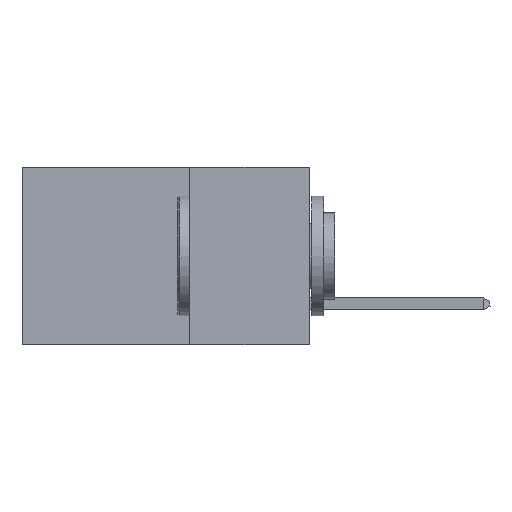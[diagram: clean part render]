
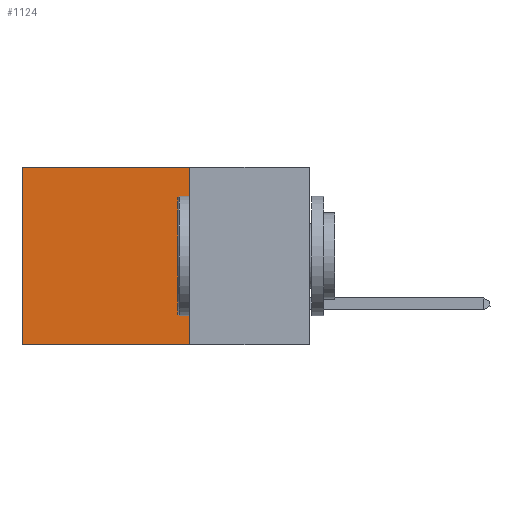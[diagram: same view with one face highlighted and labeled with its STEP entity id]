
A CAD part, left-side view. The second image highlights one B-rep face of the part: STEP entity #1124.
In plain terms, the highlighted planar face has unit normal (-1, 0, 0).
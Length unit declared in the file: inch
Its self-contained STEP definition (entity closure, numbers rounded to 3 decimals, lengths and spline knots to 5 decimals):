
#307 = DIRECTION ( 'NONE',  ( 0., 0., -1. ) ) ;
#353 = EDGE_LOOP ( 'NONE', ( #11530, #10782, #11792, #6361 ) ) ;
#507 = LINE ( 'NONE', #11734, #7460 ) ;
#599 = VERTEX_POINT ( 'NONE', #2296 ) ;
#955 = EDGE_CURVE ( 'NONE', #12459, #10195, #2803, .T. ) ;
#1124 = ADVANCED_FACE ( 'NONE', ( #12735 ), #9657, .F. ) ;
#1963 = VERTEX_POINT ( 'NONE', #11366 ) ;
#2296 = CARTESIAN_POINT ( 'NONE',  ( 0.2875, 0.25, -0.37 ) ) ;
#2623 = EDGE_CURVE ( 'NONE', #1963, #12459, #5665, .T. ) ;
#2803 = LINE ( 'NONE', #4990, #9907 ) ;
#3206 = EDGE_CURVE ( 'NONE', #599, #10195, #507, .T. ) ;
#3289 = AXIS2_PLACEMENT_3D ( 'NONE', #4396, #3425, #307 ) ;
#3303 = CARTESIAN_POINT ( 'NONE',  ( 0.2875, 0.25, 0. ) ) ;
#3425 = DIRECTION ( 'NONE',  ( 1., 0., 0. ) ) ;
#4396 = CARTESIAN_POINT ( 'NONE',  ( 0.2875, 0.25, 0. ) ) ;
#4817 = CARTESIAN_POINT ( 'NONE',  ( 0.2875, 0.6, -0.37 ) ) ;
#4990 = CARTESIAN_POINT ( 'NONE',  ( 0.2875, 0.6, 0. ) ) ;
#5665 = LINE ( 'NONE', #10748, #7131 ) ;
#5690 = DIRECTION ( 'NONE',  ( 0., 1., 0. ) ) ;
#6361 = ORIENTED_EDGE ( 'NONE', *, *, #2623, .T. ) ;
#7131 = VECTOR ( 'NONE', #5690, 39.37008 ) ;
#7460 = VECTOR ( 'NONE', #12878, 39.37008 ) ;
#7762 = CARTESIAN_POINT ( 'NONE',  ( 0.2875, 0.6, 0. ) ) ;
#9657 = PLANE ( 'NONE',  #3289 ) ;
#9907 = VECTOR ( 'NONE', #13530, 39.37008 ) ;
#10195 = VERTEX_POINT ( 'NONE', #4817 ) ;
#10344 = EDGE_CURVE ( 'NONE', #1963, #599, #11241, .T. ) ;
#10748 = CARTESIAN_POINT ( 'NONE',  ( 0.2875, 0.25, 0. ) ) ;
#10751 = DIRECTION ( 'NONE',  ( 0., 0., -1. ) ) ;
#10782 = ORIENTED_EDGE ( 'NONE', *, *, #3206, .F. ) ;
#11241 = LINE ( 'NONE', #3303, #12058 ) ;
#11366 = CARTESIAN_POINT ( 'NONE',  ( 0.2875, 0.25, 0. ) ) ;
#11530 = ORIENTED_EDGE ( 'NONE', *, *, #955, .T. ) ;
#11734 = CARTESIAN_POINT ( 'NONE',  ( 0.2875, 0.25, -0.37 ) ) ;
#11792 = ORIENTED_EDGE ( 'NONE', *, *, #10344, .F. ) ;
#12058 = VECTOR ( 'NONE', #10751, 39.37008 ) ;
#12459 = VERTEX_POINT ( 'NONE', #7762 ) ;
#12735 = FACE_OUTER_BOUND ( 'NONE', #353, .T. ) ;
#12878 = DIRECTION ( 'NONE',  ( 0., 1., 0. ) ) ;
#13530 = DIRECTION ( 'NONE',  ( 0., 0., -1. ) ) ;
